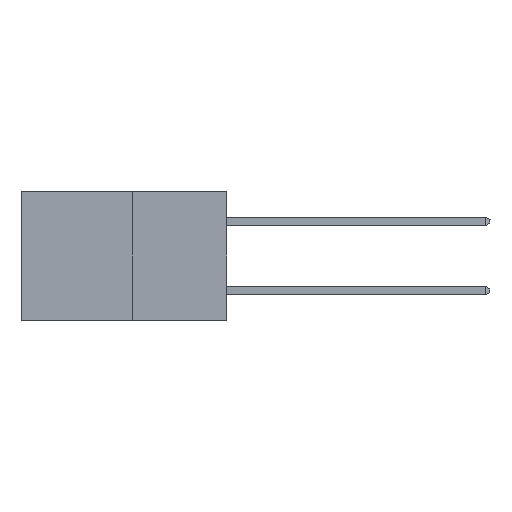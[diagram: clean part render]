
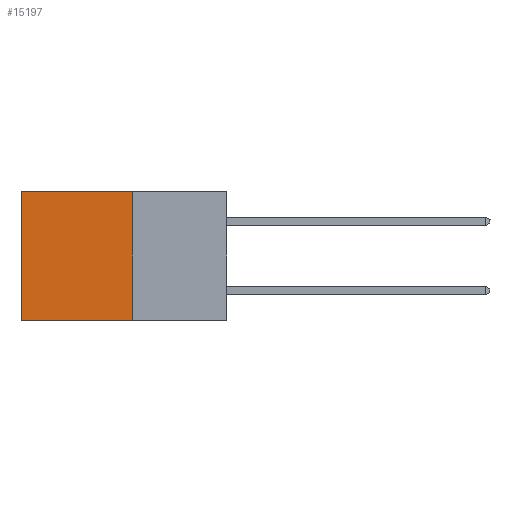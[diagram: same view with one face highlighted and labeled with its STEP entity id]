
A CAD part, left-side view. The second image highlights one B-rep face of the part: STEP entity #15197.
In plain terms, the highlighted planar face has unit normal (-1, 0, 0).
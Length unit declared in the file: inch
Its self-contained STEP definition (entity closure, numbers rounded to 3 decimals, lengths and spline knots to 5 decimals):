
#74 = VECTOR ( 'NONE', #18017, 39.37008 ) ;
#1405 = EDGE_LOOP ( 'NONE', ( #12592, #17355, #7156, #14775 ) ) ;
#2949 = FACE_OUTER_BOUND ( 'NONE', #1405, .T. ) ;
#3351 = CARTESIAN_POINT ( 'NONE',  ( 0.277, 0.59, -0.37 ) ) ;
#4035 = LINE ( 'NONE', #5434, #11045 ) ;
#4128 = DIRECTION ( 'NONE',  ( 0., 0., -1. ) ) ;
#5434 = CARTESIAN_POINT ( 'NONE',  ( 0.277, 0.27, -0.37 ) ) ;
#5575 = LINE ( 'NONE', #11712, #12588 ) ;
#5757 = VERTEX_POINT ( 'NONE', #12827 ) ;
#6390 = EDGE_CURVE ( 'NONE', #10402, #5757, #4035, .T. ) ;
#6898 = VERTEX_POINT ( 'NONE', #9956 ) ;
#7156 = ORIENTED_EDGE ( 'NONE', *, *, #6390, .F. ) ;
#7666 = LINE ( 'NONE', #3351, #74 ) ;
#7795 = EDGE_CURVE ( 'NONE', #15209, #6898, #7666, .T. ) ;
#8303 = CARTESIAN_POINT ( 'NONE',  ( 0.277, 0.59, 0. ) ) ;
#8393 = DIRECTION ( 'NONE',  ( 0., 0., -1. ) ) ;
#8711 = AXIS2_PLACEMENT_3D ( 'NONE', #9685, #12478, #4128 ) ;
#9685 = CARTESIAN_POINT ( 'NONE',  ( 0.277, 0.27, -0.37 ) ) ;
#9956 = CARTESIAN_POINT ( 'NONE',  ( 0.277, 0.59, -0.37 ) ) ;
#10402 = VERTEX_POINT ( 'NONE', #14951 ) ;
#11045 = VECTOR ( 'NONE', #8393, 39.37008 ) ;
#11102 = PLANE ( 'NONE',  #8711 ) ;
#11712 = CARTESIAN_POINT ( 'NONE',  ( 0.277, 0.27, 0. ) ) ;
#11716 = EDGE_CURVE ( 'NONE', #5757, #6898, #14652, .T. ) ;
#12478 = DIRECTION ( 'NONE',  ( 1., 0., 0. ) ) ;
#12588 = VECTOR ( 'NONE', #13038, 39.37008 ) ;
#12592 = ORIENTED_EDGE ( 'NONE', *, *, #7795, .T. ) ;
#12827 = CARTESIAN_POINT ( 'NONE',  ( 0.277, 0.27, -0.37 ) ) ;
#13038 = DIRECTION ( 'NONE',  ( 0., 1., 0. ) ) ;
#13531 = DIRECTION ( 'NONE',  ( 0., 1., 0. ) ) ;
#14222 = VECTOR ( 'NONE', #13531, 39.37008 ) ;
#14652 = LINE ( 'NONE', #17623, #14222 ) ;
#14775 = ORIENTED_EDGE ( 'NONE', *, *, #15523, .T. ) ;
#14951 = CARTESIAN_POINT ( 'NONE',  ( 0.277, 0.27, 0. ) ) ;
#15197 = ADVANCED_FACE ( 'NONE', ( #2949 ), #11102, .F. ) ;
#15209 = VERTEX_POINT ( 'NONE', #8303 ) ;
#15523 = EDGE_CURVE ( 'NONE', #10402, #15209, #5575, .T. ) ;
#17355 = ORIENTED_EDGE ( 'NONE', *, *, #11716, .F. ) ;
#17623 = CARTESIAN_POINT ( 'NONE',  ( 0.277, 0.27, -0.37 ) ) ;
#18017 = DIRECTION ( 'NONE',  ( 0., 0., -1. ) ) ;
